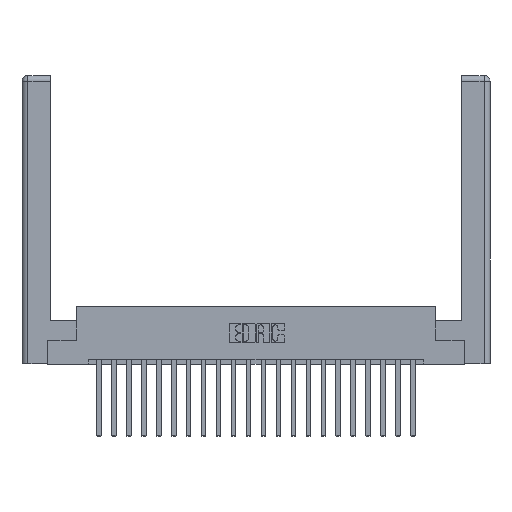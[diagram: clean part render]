
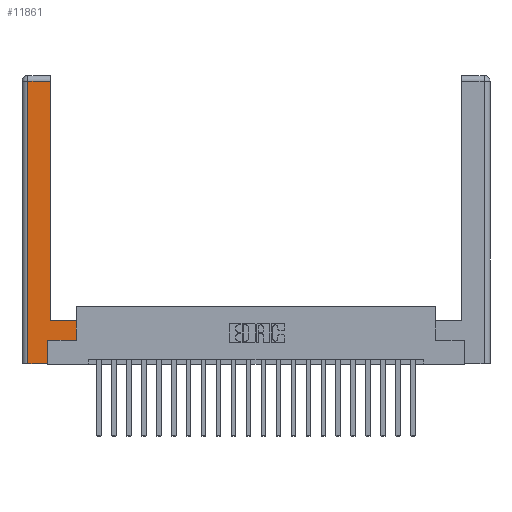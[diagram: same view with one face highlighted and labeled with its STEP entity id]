
A CAD part, top view. The second image highlights one B-rep face of the part: STEP entity #11861.
In plain terms, the highlighted planar face has unit normal (0, 0, 1).
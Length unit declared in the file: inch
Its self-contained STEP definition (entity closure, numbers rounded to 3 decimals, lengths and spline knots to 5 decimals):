
#30 = EDGE_CURVE ( 'NONE', #17884, #10267, #19486, .T. ) ;
#422 = CARTESIAN_POINT ( 'NONE',  ( 0.0615, 0., 0. ) ) ;
#602 = ORIENTED_EDGE ( 'NONE', *, *, #30, .T. ) ;
#984 = VERTEX_POINT ( 'NONE', #16487 ) ;
#1031 = LINE ( 'NONE', #11697, #13526 ) ;
#1304 = ORIENTED_EDGE ( 'NONE', *, *, #15779, .T. ) ;
#1454 = EDGE_LOOP ( 'NONE', ( #6617, #15459, #5996, #602, #16948, #5616, #1304, #22049 ) ) ;
#1509 = DIRECTION ( 'NONE',  ( 0., 1., 0. ) ) ;
#1896 = VECTOR ( 'NONE', #17010, 39.37008 ) ;
#2235 = DIRECTION ( 'NONE',  ( 0., 1., 0. ) ) ;
#2464 = EDGE_CURVE ( 'NONE', #20174, #3737, #2858, .T. ) ;
#2858 = LINE ( 'NONE', #5196, #3385 ) ;
#3021 = VECTOR ( 'NONE', #5370, 39.37008 ) ;
#3287 = LINE ( 'NONE', #19027, #3021 ) ;
#3385 = VECTOR ( 'NONE', #13716, 39.37008 ) ;
#3468 = EDGE_CURVE ( 'NONE', #10267, #20174, #6784, .T. ) ;
#3737 = VERTEX_POINT ( 'NONE', #5493 ) ;
#4314 = CARTESIAN_POINT ( 'NONE',  ( 0.265, 0.245, 0. ) ) ;
#4711 = EDGE_CURVE ( 'NONE', #20171, #15647, #5293, .T. ) ;
#5103 = VECTOR ( 'NONE', #7425, 39.37008 ) ;
#5196 = CARTESIAN_POINT ( 'NONE',  ( 0.565, 0.245, 0. ) ) ;
#5293 = LINE ( 'NONE', #12572, #7663 ) ;
#5370 = DIRECTION ( 'NONE',  ( 0., -1., 0. ) ) ;
#5493 = CARTESIAN_POINT ( 'NONE',  ( 0.565, 0.245, 0. ) ) ;
#5590 = AXIS2_PLACEMENT_3D ( 'NONE', #16281, #9567, #13070 ) ;
#5616 = ORIENTED_EDGE ( 'NONE', *, *, #2464, .T. ) ;
#5996 = ORIENTED_EDGE ( 'NONE', *, *, #17840, .T. ) ;
#6617 = ORIENTED_EDGE ( 'NONE', *, *, #4711, .T. ) ;
#6784 = LINE ( 'NONE', #4314, #15330 ) ;
#7425 = DIRECTION ( 'NONE',  ( -1., 0., 0. ) ) ;
#7663 = VECTOR ( 'NONE', #2235, 39.37008 ) ;
#8056 = DIRECTION ( 'NONE',  ( 1., 0., 0. ) ) ;
#8127 = CARTESIAN_POINT ( 'NONE',  ( 0.265, 0., 0. ) ) ;
#8343 = CARTESIAN_POINT ( 'NONE',  ( 0.0615, 2.94, 0. ) ) ;
#9144 = FACE_OUTER_BOUND ( 'NONE', #1454, .T. ) ;
#9567 = DIRECTION ( 'NONE',  ( 0., 0., -1. ) ) ;
#10267 = VERTEX_POINT ( 'NONE', #13672 ) ;
#10910 = DIRECTION ( 'NONE',  ( 0., 1., 0. ) ) ;
#11459 = LINE ( 'NONE', #15935, #5103 ) ;
#11697 = CARTESIAN_POINT ( 'NONE',  ( 0.565, 0.45, 0. ) ) ;
#11755 = CARTESIAN_POINT ( 'NONE',  ( 0.295, 0.45, 0. ) ) ;
#11861 = ADVANCED_FACE ( 'NONE', ( #9144 ), #21672, .F. ) ;
#12016 = LINE ( 'NONE', #8343, #1896 ) ;
#12250 = VECTOR ( 'NONE', #8056, 39.37008 ) ;
#12572 = CARTESIAN_POINT ( 'NONE',  ( 0.295, 3., 0. ) ) ;
#12981 = CARTESIAN_POINT ( 'NONE',  ( 0.0615, 2.94, 0. ) ) ;
#13070 = DIRECTION ( 'NONE',  ( -1., 0., 0. ) ) ;
#13132 = CARTESIAN_POINT ( 'NONE',  ( 0.295, 2.94, 0. ) ) ;
#13252 = CARTESIAN_POINT ( 'NONE',  ( 0.265, 0.245, 0. ) ) ;
#13526 = VECTOR ( 'NONE', #1509, 39.37008 ) ;
#13672 = CARTESIAN_POINT ( 'NONE',  ( 0.265, 0., 0. ) ) ;
#13716 = DIRECTION ( 'NONE',  ( 1., 0., 0. ) ) ;
#15330 = VECTOR ( 'NONE', #10910, 39.37008 ) ;
#15459 = ORIENTED_EDGE ( 'NONE', *, *, #18926, .T. ) ;
#15647 = VERTEX_POINT ( 'NONE', #13132 ) ;
#15779 = EDGE_CURVE ( 'NONE', #3737, #984, #1031, .T. ) ;
#15935 = CARTESIAN_POINT ( 'NONE',  ( 0.295, 0.45, 0. ) ) ;
#16281 = CARTESIAN_POINT ( 'NONE',  ( 0., 0., 0. ) ) ;
#16487 = CARTESIAN_POINT ( 'NONE',  ( 0.565, 0.45, 0. ) ) ;
#16948 = ORIENTED_EDGE ( 'NONE', *, *, #3468, .T. ) ;
#17010 = DIRECTION ( 'NONE',  ( -1., 0., 0. ) ) ;
#17840 = EDGE_CURVE ( 'NONE', #18810, #17884, #3287, .T. ) ;
#17884 = VERTEX_POINT ( 'NONE', #422 ) ;
#18810 = VERTEX_POINT ( 'NONE', #12981 ) ;
#18926 = EDGE_CURVE ( 'NONE', #15647, #18810, #12016, .T. ) ;
#19027 = CARTESIAN_POINT ( 'NONE',  ( 0.0615, 0., 0. ) ) ;
#19286 = EDGE_CURVE ( 'NONE', #984, #20171, #11459, .T. ) ;
#19486 = LINE ( 'NONE', #8127, #12250 ) ;
#20171 = VERTEX_POINT ( 'NONE', #11755 ) ;
#20174 = VERTEX_POINT ( 'NONE', #13252 ) ;
#21672 = PLANE ( 'NONE',  #5590 ) ;
#22049 = ORIENTED_EDGE ( 'NONE', *, *, #19286, .T. ) ;
